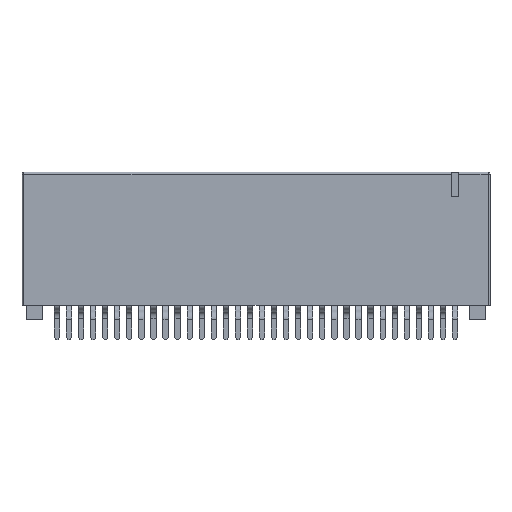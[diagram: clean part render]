
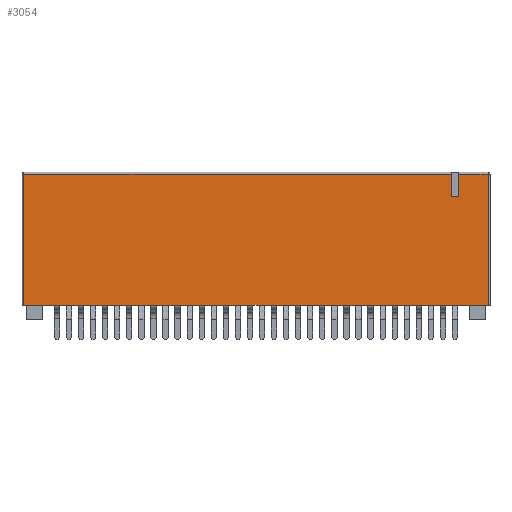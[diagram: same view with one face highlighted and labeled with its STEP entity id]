
A CAD part, top view. The second image highlights one B-rep face of the part: STEP entity #3054.
In plain terms, the highlighted planar face has unit normal (0, 0, 1).
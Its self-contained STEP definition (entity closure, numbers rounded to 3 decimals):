
#892 = VERTEX_POINT ( 'NONE', #11446 ) ;
#948 = VERTEX_POINT ( 'NONE', #22330 ) ;
#1097 = LINE ( 'NONE', #27802, #2322 ) ;
#1233 = CARTESIAN_POINT ( 'NONE',  ( 0.2, 15.5, 0. ) ) ;
#1400 = LINE ( 'NONE', #25549, #25889 ) ;
#1674 = CARTESIAN_POINT ( 'NONE',  ( 0., 15.5, 0. ) ) ;
#1686 = VECTOR ( 'NONE', #19409, 1000. ) ;
#2322 = VECTOR ( 'NONE', #8214, 1000. ) ;
#2478 = CARTESIAN_POINT ( 'NONE',  ( 45.985, 12.95, 0. ) ) ;
#2574 = VECTOR ( 'NONE', #8294, 1000. ) ;
#3054 = ADVANCED_FACE ( 'NONE', ( #23409 ), #21259, .F. ) ;
#3398 = DIRECTION ( 'NONE',  ( -1., 0., 0. ) ) ;
#4408 = ORIENTED_EDGE ( 'NONE', *, *, #22746, .T. ) ;
#6094 = DIRECTION ( 'NONE',  ( 0., 0., -1. ) ) ;
#6152 = ORIENTED_EDGE ( 'NONE', *, *, #18436, .F. ) ;
#7175 = EDGE_CURVE ( 'NONE', #24449, #7268, #1097, .T. ) ;
#7268 = VERTEX_POINT ( 'NONE', #19682 ) ;
#8208 = CARTESIAN_POINT ( 'NONE',  ( 0.2, 1.5, 0. ) ) ;
#8214 = DIRECTION ( 'NONE',  ( -1., 0., 0. ) ) ;
#8294 = DIRECTION ( 'NONE',  ( 1., 0., 0. ) ) ;
#8400 = VERTEX_POINT ( 'NONE', #24123 ) ;
#9022 = VECTOR ( 'NONE', #18877, 1000. ) ;
#9302 = DIRECTION ( 'NONE',  ( 0., 1., 0. ) ) ;
#9440 = CARTESIAN_POINT ( 'NONE',  ( 49.08, 15.3, 0. ) ) ;
#10150 = LINE ( 'NONE', #21607, #2574 ) ;
#10816 = LINE ( 'NONE', #23416, #1686 ) ;
#11050 = LINE ( 'NONE', #2478, #22706 ) ;
#11446 = CARTESIAN_POINT ( 'NONE',  ( 45.205, 12.95, 0. ) ) ;
#12106 = CARTESIAN_POINT ( 'NONE',  ( 0., 15.3, 0. ) ) ;
#12302 = EDGE_LOOP ( 'NONE', ( #19918, #18963, #17003, #20785, #6152, #4408, #28198, #22292 ) ) ;
#14238 = LINE ( 'NONE', #1233, #18677 ) ;
#15639 = DIRECTION ( 'NONE',  ( 0., 1., 0. ) ) ;
#16143 = LINE ( 'NONE', #12106, #19922 ) ;
#16338 = EDGE_CURVE ( 'NONE', #948, #22174, #11050, .T. ) ;
#16947 = EDGE_CURVE ( 'NONE', #21327, #22174, #16143, .T. ) ;
#17003 = ORIENTED_EDGE ( 'NONE', *, *, #7175, .T. ) ;
#18236 = EDGE_CURVE ( 'NONE', #892, #24449, #1400, .T. ) ;
#18436 = EDGE_CURVE ( 'NONE', #8400, #25104, #10816, .T. ) ;
#18677 = VECTOR ( 'NONE', #22694, 1000. ) ;
#18877 = DIRECTION ( 'NONE',  ( 0., 1., 0. ) ) ;
#18963 = ORIENTED_EDGE ( 'NONE', *, *, #18236, .T. ) ;
#19409 = DIRECTION ( 'NONE',  ( -1., 0., 0. ) ) ;
#19682 = CARTESIAN_POINT ( 'NONE',  ( 0.2, 15.3, 0. ) ) ;
#19918 = ORIENTED_EDGE ( 'NONE', *, *, #21079, .F. ) ;
#19922 = VECTOR ( 'NONE', #3398, 1000. ) ;
#20785 = ORIENTED_EDGE ( 'NONE', *, *, #25024, .T. ) ;
#21021 = CARTESIAN_POINT ( 'NONE',  ( 49.08, 15.5, 0. ) ) ;
#21079 = EDGE_CURVE ( 'NONE', #892, #948, #10150, .T. ) ;
#21259 = PLANE ( 'NONE',  #25786 ) ;
#21327 = VERTEX_POINT ( 'NONE', #9440 ) ;
#21607 = CARTESIAN_POINT ( 'NONE',  ( 45.205, 12.95, 0. ) ) ;
#22174 = VERTEX_POINT ( 'NONE', #24398 ) ;
#22292 = ORIENTED_EDGE ( 'NONE', *, *, #16338, .F. ) ;
#22330 = CARTESIAN_POINT ( 'NONE',  ( 45.985, 12.95, 0. ) ) ;
#22694 = DIRECTION ( 'NONE',  ( 0., -1., 0. ) ) ;
#22706 = VECTOR ( 'NONE', #15639, 1000. ) ;
#22746 = EDGE_CURVE ( 'NONE', #8400, #21327, #27297, .T. ) ;
#23409 = FACE_OUTER_BOUND ( 'NONE', #12302, .T. ) ;
#23416 = CARTESIAN_POINT ( 'NONE',  ( 49.28, 1.5, 0. ) ) ;
#23548 = DIRECTION ( 'NONE',  ( -1., 0., 0. ) ) ;
#24123 = CARTESIAN_POINT ( 'NONE',  ( 49.08, 1.5, 0. ) ) ;
#24398 = CARTESIAN_POINT ( 'NONE',  ( 45.985, 15.3, 0. ) ) ;
#24449 = VERTEX_POINT ( 'NONE', #25169 ) ;
#25024 = EDGE_CURVE ( 'NONE', #7268, #25104, #14238, .T. ) ;
#25104 = VERTEX_POINT ( 'NONE', #8208 ) ;
#25169 = CARTESIAN_POINT ( 'NONE',  ( 45.205, 15.3, 0. ) ) ;
#25549 = CARTESIAN_POINT ( 'NONE',  ( 45.205, 12.95, 0. ) ) ;
#25786 = AXIS2_PLACEMENT_3D ( 'NONE', #1674, #6094, #23548 ) ;
#25889 = VECTOR ( 'NONE', #9302, 1000. ) ;
#27297 = LINE ( 'NONE', #21021, #9022 ) ;
#27802 = CARTESIAN_POINT ( 'NONE',  ( 0., 15.3, 0. ) ) ;
#28198 = ORIENTED_EDGE ( 'NONE', *, *, #16947, .T. ) ;
